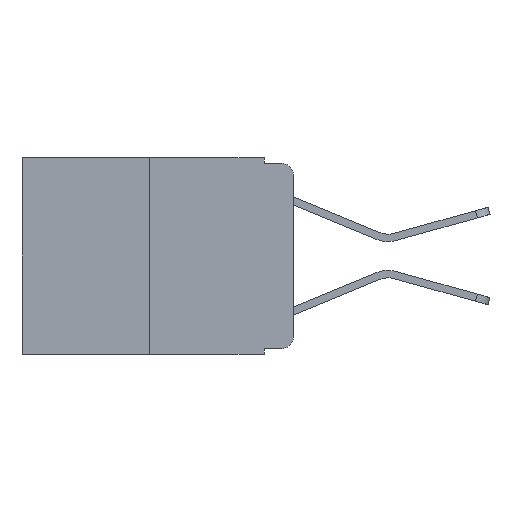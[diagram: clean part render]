
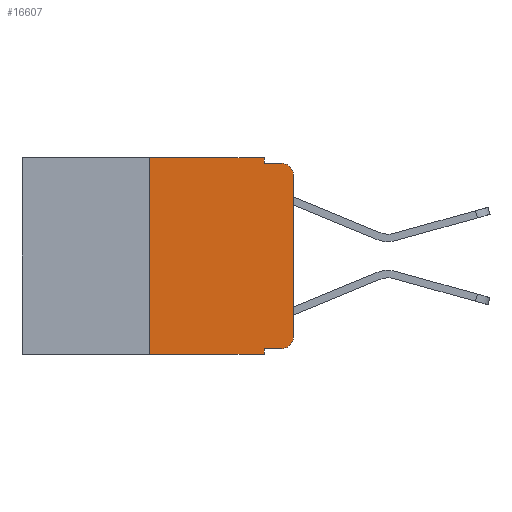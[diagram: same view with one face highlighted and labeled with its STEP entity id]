
A CAD part, left-side view. The second image highlights one B-rep face of the part: STEP entity #16607.
In plain terms, the highlighted planar face has unit normal (-1, 0, 0).
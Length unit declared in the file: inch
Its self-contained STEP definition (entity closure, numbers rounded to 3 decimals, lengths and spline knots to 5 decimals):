
#61 = VERTEX_POINT ( 'NONE', #15208 ) ;
#102 = VERTEX_POINT ( 'NONE', #18283 ) ;
#302 = EDGE_CURVE ( 'NONE', #102, #13352, #5242, .T. ) ;
#626 = AXIS2_PLACEMENT_3D ( 'NONE', #2364, #14102, #10954 ) ;
#826 = LINE ( 'NONE', #18902, #18275 ) ;
#994 = EDGE_LOOP ( 'NONE', ( #4145, #4344, #15721, #16474, #2610, #2668, #18823, #19334, #4420, #3229 ) ) ;
#1285 = DIRECTION ( 'NONE',  ( 0., -1., 0. ) ) ;
#1675 = EDGE_CURVE ( 'NONE', #11140, #61, #2306, .T. ) ;
#1888 = VECTOR ( 'NONE', #11744, 39.37008 ) ;
#1980 = DIRECTION ( 'NONE',  ( 0., 0., 1. ) ) ;
#2306 = LINE ( 'NONE', #11397, #9050 ) ;
#2364 = CARTESIAN_POINT ( 'NONE',  ( 0., 0.473, 0. ) ) ;
#2536 = CIRCLE ( 'NONE', #13552, 0.02 ) ;
#2610 = ORIENTED_EDGE ( 'NONE', *, *, #14178, .F. ) ;
#2668 = ORIENTED_EDGE ( 'NONE', *, *, #4186, .F. ) ;
#2948 = DIRECTION ( 'NONE',  ( -1., 0., 0. ) ) ;
#3229 = ORIENTED_EDGE ( 'NONE', *, *, #3485, .T. ) ;
#3485 = EDGE_CURVE ( 'NONE', #4142, #102, #13896, .T. ) ;
#3529 = LINE ( 'NONE', #15466, #16125 ) ;
#3534 = DIRECTION ( 'NONE',  ( 0., -1., 0. ) ) ;
#3617 = VECTOR ( 'NONE', #13540, 39.37008 ) ;
#3762 = CARTESIAN_POINT ( 'NONE',  ( 0., 0.051, -0.343 ) ) ;
#3785 = DIRECTION ( 'NONE',  ( 0., -1., 0. ) ) ;
#4142 = VERTEX_POINT ( 'NONE', #18529 ) ;
#4145 = ORIENTED_EDGE ( 'NONE', *, *, #302, .T. ) ;
#4186 = EDGE_CURVE ( 'NONE', #4498, #15472, #18629, .T. ) ;
#4344 = ORIENTED_EDGE ( 'NONE', *, *, #9926, .T. ) ;
#4420 = ORIENTED_EDGE ( 'NONE', *, *, #9224, .T. ) ;
#4498 = VERTEX_POINT ( 'NONE', #18215 ) ;
#4592 = VECTOR ( 'NONE', #3534, 39.37008 ) ;
#4635 = DIRECTION ( 'NONE',  ( 0., 0., -1. ) ) ;
#4716 = CARTESIAN_POINT ( 'NONE',  ( 0., 0.473, -0.343 ) ) ;
#5242 = LINE ( 'NONE', #6819, #13581 ) ;
#5394 = AXIS2_PLACEMENT_3D ( 'NONE', #16466, #2948, #5890 ) ;
#5890 = DIRECTION ( 'NONE',  ( 0., 0., -1. ) ) ;
#6239 = CARTESIAN_POINT ( 'NONE',  ( 0., 0.25, 0. ) ) ;
#6783 = EDGE_CURVE ( 'NONE', #4498, #9754, #7679, .T. ) ;
#6819 = CARTESIAN_POINT ( 'NONE',  ( 0., 0., 0. ) ) ;
#7369 = VERTEX_POINT ( 'NONE', #11755 ) ;
#7563 = VECTOR ( 'NONE', #9541, 39.37008 ) ;
#7679 = LINE ( 'NONE', #4716, #4592 ) ;
#7985 = FACE_OUTER_BOUND ( 'NONE', #994, .T. ) ;
#9050 = VECTOR ( 'NONE', #1285, 39.37008 ) ;
#9224 = EDGE_CURVE ( 'NONE', #7369, #4142, #826, .T. ) ;
#9541 = DIRECTION ( 'NONE',  ( 0., 0., 1. ) ) ;
#9754 = VERTEX_POINT ( 'NONE', #3762 ) ;
#9870 = EDGE_CURVE ( 'NONE', #18959, #11140, #11645, .T. ) ;
#9926 = EDGE_CURVE ( 'NONE', #13352, #61, #2536, .T. ) ;
#9978 = CARTESIAN_POINT ( 'NONE',  ( 0., 0.051, 0. ) ) ;
#10954 = DIRECTION ( 'NONE',  ( 0., 0., -1. ) ) ;
#11140 = VERTEX_POINT ( 'NONE', #15433 ) ;
#11397 = CARTESIAN_POINT ( 'NONE',  ( 0., 0.051, -0.01 ) ) ;
#11645 = LINE ( 'NONE', #9978, #1888 ) ;
#11744 = DIRECTION ( 'NONE',  ( 0., 0., -1. ) ) ;
#11755 = CARTESIAN_POINT ( 'NONE',  ( 0., 0.051, -0.333 ) ) ;
#11853 = DIRECTION ( 'NONE',  ( -1., 0., 0. ) ) ;
#11978 = LINE ( 'NONE', #16703, #3617 ) ;
#13352 = VERTEX_POINT ( 'NONE', #13784 ) ;
#13540 = DIRECTION ( 'NONE',  ( 0., -1., 0. ) ) ;
#13552 = AXIS2_PLACEMENT_3D ( 'NONE', #18269, #11853, #4635 ) ;
#13581 = VECTOR ( 'NONE', #1980, 39.37008 ) ;
#13784 = CARTESIAN_POINT ( 'NONE',  ( 0., 0., -0.03 ) ) ;
#13896 = CIRCLE ( 'NONE', #5394, 0.02 ) ;
#13999 = PLANE ( 'NONE',  #626 ) ;
#14102 = DIRECTION ( 'NONE',  ( 1., 0., 0. ) ) ;
#14178 = EDGE_CURVE ( 'NONE', #15472, #18959, #11978, .T. ) ;
#14452 = CARTESIAN_POINT ( 'NONE',  ( 0., 0.051, 0. ) ) ;
#15208 = CARTESIAN_POINT ( 'NONE',  ( 0., 0.02, -0.01 ) ) ;
#15433 = CARTESIAN_POINT ( 'NONE',  ( 0., 0.051, -0.01 ) ) ;
#15466 = CARTESIAN_POINT ( 'NONE',  ( 0., 0.051, 0. ) ) ;
#15472 = VERTEX_POINT ( 'NONE', #6239 ) ;
#15721 = ORIENTED_EDGE ( 'NONE', *, *, #1675, .F. ) ;
#16125 = VECTOR ( 'NONE', #18742, 39.37008 ) ;
#16466 = CARTESIAN_POINT ( 'NONE',  ( 0., 0.02, -0.313 ) ) ;
#16474 = ORIENTED_EDGE ( 'NONE', *, *, #9870, .F. ) ;
#16607 = ADVANCED_FACE ( 'NONE', ( #7985 ), #13999, .F. ) ;
#16703 = CARTESIAN_POINT ( 'NONE',  ( 0., 0.473, 0. ) ) ;
#18215 = CARTESIAN_POINT ( 'NONE',  ( 0., 0.25, -0.343 ) ) ;
#18235 = CARTESIAN_POINT ( 'NONE',  ( 0., 0.25, 0. ) ) ;
#18269 = CARTESIAN_POINT ( 'NONE',  ( 0., 0.02, -0.03 ) ) ;
#18275 = VECTOR ( 'NONE', #3785, 39.37008 ) ;
#18283 = CARTESIAN_POINT ( 'NONE',  ( 0., 0., -0.313 ) ) ;
#18411 = EDGE_CURVE ( 'NONE', #7369, #9754, #3529, .T. ) ;
#18529 = CARTESIAN_POINT ( 'NONE',  ( 0., 0.02, -0.333 ) ) ;
#18629 = LINE ( 'NONE', #18235, #7563 ) ;
#18742 = DIRECTION ( 'NONE',  ( 0., 0., -1. ) ) ;
#18823 = ORIENTED_EDGE ( 'NONE', *, *, #6783, .T. ) ;
#18902 = CARTESIAN_POINT ( 'NONE',  ( 0., 0.051, -0.333 ) ) ;
#18959 = VERTEX_POINT ( 'NONE', #14452 ) ;
#19334 = ORIENTED_EDGE ( 'NONE', *, *, #18411, .F. ) ;
